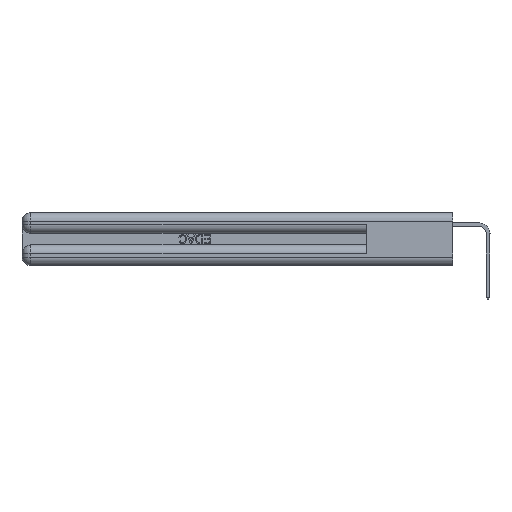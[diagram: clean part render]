
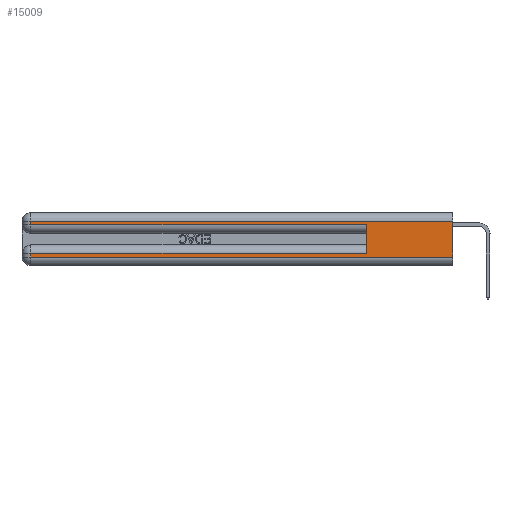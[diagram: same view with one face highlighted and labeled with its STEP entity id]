
A CAD part, left-side view. The second image highlights one B-rep face of the part: STEP entity #15009.
In plain terms, the highlighted planar face has unit normal (-1, 0, 0).
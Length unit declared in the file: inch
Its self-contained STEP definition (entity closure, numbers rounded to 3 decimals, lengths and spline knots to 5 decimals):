
#49 = EDGE_CURVE ( 'NONE', #22893, #21375, #31906, .T. ) ;
#61 = ORIENTED_EDGE ( 'NONE', *, *, #1050, .T. ) ;
#779 = CARTESIAN_POINT ( 'NONE',  ( 0., 0.6, 0.145 ) ) ;
#933 = DIRECTION ( 'NONE',  ( 0., 0., 1. ) ) ;
#986 = VERTEX_POINT ( 'NONE', #11043 ) ;
#1050 = EDGE_CURVE ( 'NONE', #29117, #24090, #13874, .T. ) ;
#1781 = VERTEX_POINT ( 'NONE', #36563 ) ;
#3224 = ORIENTED_EDGE ( 'NONE', *, *, #38127, .T. ) ;
#3698 = CARTESIAN_POINT ( 'NONE',  ( 0., 0., 0.31 ) ) ;
#4505 = EDGE_CURVE ( 'NONE', #9239, #6564, #27335, .T. ) ;
#4879 = LINE ( 'NONE', #35338, #12813 ) ;
#5018 = ORIENTED_EDGE ( 'NONE', *, *, #26474, .T. ) ;
#6564 = VERTEX_POINT ( 'NONE', #27640 ) ;
#9239 = VERTEX_POINT ( 'NONE', #36263 ) ;
#9978 = DIRECTION ( 'NONE',  ( 0., 0., -1. ) ) ;
#11043 = CARTESIAN_POINT ( 'NONE',  ( 0., 2.94, 0.31 ) ) ;
#11100 = ORIENTED_EDGE ( 'NONE', *, *, #49, .F. ) ;
#11417 = LINE ( 'NONE', #31934, #19344 ) ;
#12804 = VECTOR ( 'NONE', #39256, 39.37008 ) ;
#12813 = VECTOR ( 'NONE', #32122, 39.37008 ) ;
#12933 = CARTESIAN_POINT ( 'NONE',  ( 0., 2.94, 0.06 ) ) ;
#13337 = DIRECTION ( 'NONE',  ( 0., -1., 0. ) ) ;
#13874 = LINE ( 'NONE', #36053, #12804 ) ;
#14053 = EDGE_CURVE ( 'NONE', #1781, #29117, #11417, .T. ) ;
#14508 = FACE_OUTER_BOUND ( 'NONE', #20319, .T. ) ;
#15009 = ADVANCED_FACE ( 'NONE', ( #14508 ), #23422, .F. ) ;
#15128 = DIRECTION ( 'NONE',  ( 0., 1., 0. ) ) ;
#19107 = ORIENTED_EDGE ( 'NONE', *, *, #41558, .T. ) ;
#19344 = VECTOR ( 'NONE', #15128, 39.37008 ) ;
#19420 = LINE ( 'NONE', #36613, #34182 ) ;
#19818 = DIRECTION ( 'NONE',  ( 0., 1., 0. ) ) ;
#20319 = EDGE_LOOP ( 'NONE', ( #11100, #19107, #5018, #27620, #22543, #28949, #61, #3224 ) ) ;
#20455 = VECTOR ( 'NONE', #13337, 39.37008 ) ;
#21375 = VERTEX_POINT ( 'NONE', #28351 ) ;
#21874 = VECTOR ( 'NONE', #42616, 39.37008 ) ;
#22543 = ORIENTED_EDGE ( 'NONE', *, *, #28613, .F. ) ;
#22893 = VERTEX_POINT ( 'NONE', #3698 ) ;
#23422 = PLANE ( 'NONE',  #29715 ) ;
#23922 = CARTESIAN_POINT ( 'NONE',  ( 0., 2.94, 0.085 ) ) ;
#24090 = VERTEX_POINT ( 'NONE', #12933 ) ;
#25903 = CARTESIAN_POINT ( 'NONE',  ( 0., 0., 0.37 ) ) ;
#26474 = EDGE_CURVE ( 'NONE', #986, #9239, #27354, .T. ) ;
#26687 = CARTESIAN_POINT ( 'NONE',  ( 0., 0., 0.37 ) ) ;
#27335 = LINE ( 'NONE', #33537, #20455 ) ;
#27354 = LINE ( 'NONE', #29544, #35245 ) ;
#27620 = ORIENTED_EDGE ( 'NONE', *, *, #4505, .T. ) ;
#27640 = CARTESIAN_POINT ( 'NONE',  ( 0., 0.6, 0.285 ) ) ;
#28220 = VECTOR ( 'NONE', #933, 39.37008 ) ;
#28351 = CARTESIAN_POINT ( 'NONE',  ( 0., 0., 0.06 ) ) ;
#28613 = EDGE_CURVE ( 'NONE', #1781, #6564, #38174, .T. ) ;
#28949 = ORIENTED_EDGE ( 'NONE', *, *, #14053, .T. ) ;
#29117 = VERTEX_POINT ( 'NONE', #23922 ) ;
#29544 = CARTESIAN_POINT ( 'NONE',  ( 0., 2.94, 0.37 ) ) ;
#29715 = AXIS2_PLACEMENT_3D ( 'NONE', #26687, #30216, #9978 ) ;
#30216 = DIRECTION ( 'NONE',  ( 1., 0., 0. ) ) ;
#31906 = LINE ( 'NONE', #25903, #21874 ) ;
#31934 = CARTESIAN_POINT ( 'NONE',  ( 0., 0., 0.085 ) ) ;
#32122 = DIRECTION ( 'NONE',  ( 0., -1., 0. ) ) ;
#33537 = CARTESIAN_POINT ( 'NONE',  ( 0., 0., 0.285 ) ) ;
#34182 = VECTOR ( 'NONE', #19818, 39.37008 ) ;
#35245 = VECTOR ( 'NONE', #36306, 39.37008 ) ;
#35338 = CARTESIAN_POINT ( 'NONE',  ( 0., 0., 0.06 ) ) ;
#36053 = CARTESIAN_POINT ( 'NONE',  ( 0., 2.94, 0.37 ) ) ;
#36263 = CARTESIAN_POINT ( 'NONE',  ( 0., 2.94, 0.285 ) ) ;
#36306 = DIRECTION ( 'NONE',  ( 0., 0., -1. ) ) ;
#36563 = CARTESIAN_POINT ( 'NONE',  ( 0., 0.6, 0.085 ) ) ;
#36613 = CARTESIAN_POINT ( 'NONE',  ( 0., 0., 0.31 ) ) ;
#38127 = EDGE_CURVE ( 'NONE', #24090, #21375, #4879, .T. ) ;
#38174 = LINE ( 'NONE', #779, #28220 ) ;
#39256 = DIRECTION ( 'NONE',  ( 0., 0., -1. ) ) ;
#41558 = EDGE_CURVE ( 'NONE', #22893, #986, #19420, .T. ) ;
#42616 = DIRECTION ( 'NONE',  ( 0., 0., -1. ) ) ;
